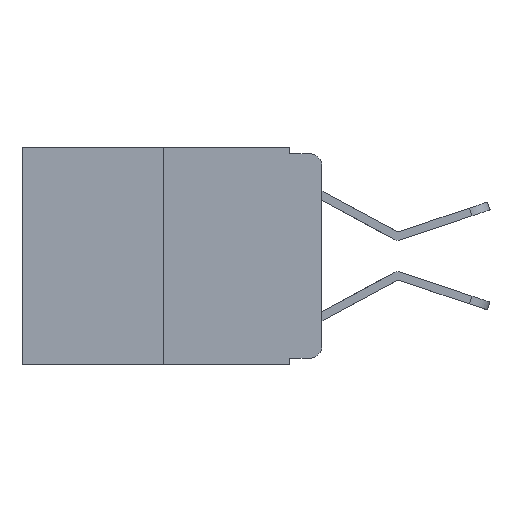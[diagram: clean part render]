
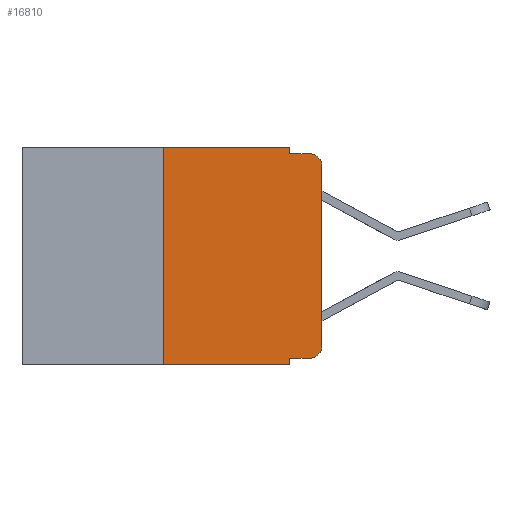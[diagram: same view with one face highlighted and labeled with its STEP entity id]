
A CAD part, left-side view. The second image highlights one B-rep face of the part: STEP entity #16810.
In plain terms, the highlighted planar face has unit normal (-1, 0, 0).
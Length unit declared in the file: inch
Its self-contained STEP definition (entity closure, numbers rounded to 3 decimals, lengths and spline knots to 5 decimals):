
#11 = EDGE_CURVE ( 'NONE', #2553, #739, #17145, .T. ) ;
#64 = ORIENTED_EDGE ( 'NONE', *, *, #16250, .F. ) ;
#450 = EDGE_CURVE ( 'NONE', #16306, #8936, #7758, .T. ) ;
#457 = CARTESIAN_POINT ( 'NONE',  ( 0., 0.02, -0.333 ) ) ;
#739 = VERTEX_POINT ( 'NONE', #10599 ) ;
#874 = CARTESIAN_POINT ( 'NONE',  ( 0., 0.473, -0.343 ) ) ;
#1337 = DIRECTION ( 'NONE',  ( 0., 0., 1. ) ) ;
#1581 = CARTESIAN_POINT ( 'NONE',  ( 0., 0.02, -0.313 ) ) ;
#1829 = EDGE_CURVE ( 'NONE', #11081, #2553, #3746, .T. ) ;
#2377 = PLANE ( 'NONE',  #7159 ) ;
#2470 = CARTESIAN_POINT ( 'NONE',  ( 0., 0.25, -0.343 ) ) ;
#2553 = VERTEX_POINT ( 'NONE', #6418 ) ;
#2650 = DIRECTION ( 'NONE',  ( 0., -1., 0. ) ) ;
#2667 = DIRECTION ( 'NONE',  ( 0., 0., -1. ) ) ;
#2817 = VERTEX_POINT ( 'NONE', #11243 ) ;
#3162 = VERTEX_POINT ( 'NONE', #4280 ) ;
#3557 = VERTEX_POINT ( 'NONE', #457 ) ;
#3746 = LINE ( 'NONE', #15966, #10415 ) ;
#3912 = CARTESIAN_POINT ( 'NONE',  ( 0., 0.473, 0. ) ) ;
#3955 = DIRECTION ( 'NONE',  ( 0., 0., -1. ) ) ;
#4280 = CARTESIAN_POINT ( 'NONE',  ( 0., 0.051, -0.343 ) ) ;
#4522 = VECTOR ( 'NONE', #1337, 39.37008 ) ;
#4531 = ORIENTED_EDGE ( 'NONE', *, *, #12968, .T. ) ;
#4738 = CIRCLE ( 'NONE', #11018, 0.02 ) ;
#5522 = CARTESIAN_POINT ( 'NONE',  ( 0., 0.051, 0. ) ) ;
#5604 = CARTESIAN_POINT ( 'NONE',  ( 0., 0., -0.313 ) ) ;
#5873 = DIRECTION ( 'NONE',  ( 0., 0., -1. ) ) ;
#5880 = DIRECTION ( 'NONE',  ( 0., 0., 1. ) ) ;
#5907 = DIRECTION ( 'NONE',  ( -1., 0., 0. ) ) ;
#6418 = CARTESIAN_POINT ( 'NONE',  ( 0., 0., -0.03 ) ) ;
#6440 = VECTOR ( 'NONE', #13638, 39.37008 ) ;
#6793 = EDGE_CURVE ( 'NONE', #2817, #3557, #14821, .T. ) ;
#6805 = ORIENTED_EDGE ( 'NONE', *, *, #10456, .F. ) ;
#7011 = EDGE_CURVE ( 'NONE', #8936, #14235, #13472, .T. ) ;
#7159 = AXIS2_PLACEMENT_3D ( 'NONE', #14167, #12727, #3955 ) ;
#7430 = ORIENTED_EDGE ( 'NONE', *, *, #7011, .F. ) ;
#7619 = CARTESIAN_POINT ( 'NONE',  ( 0., 0.051, 0. ) ) ;
#7758 = LINE ( 'NONE', #3912, #12862 ) ;
#8413 = CARTESIAN_POINT ( 'NONE',  ( 0., 0.25, 0. ) ) ;
#8647 = VECTOR ( 'NONE', #9802, 39.37008 ) ;
#8850 = CARTESIAN_POINT ( 'NONE',  ( 0., 0.25, 0. ) ) ;
#8936 = VERTEX_POINT ( 'NONE', #16142 ) ;
#8995 = ORIENTED_EDGE ( 'NONE', *, *, #450, .F. ) ;
#9296 = ORIENTED_EDGE ( 'NONE', *, *, #6793, .T. ) ;
#9513 = FACE_OUTER_BOUND ( 'NONE', #14394, .T. ) ;
#9802 = DIRECTION ( 'NONE',  ( 0., -1., 0. ) ) ;
#9856 = ORIENTED_EDGE ( 'NONE', *, *, #14492, .F. ) ;
#10194 = DIRECTION ( 'NONE',  ( 0., 0., -1. ) ) ;
#10196 = VECTOR ( 'NONE', #2667, 39.37008 ) ;
#10212 = VECTOR ( 'NONE', #10510, 39.37008 ) ;
#10415 = VECTOR ( 'NONE', #5880, 39.37008 ) ;
#10456 = EDGE_CURVE ( 'NONE', #16120, #16306, #14461, .T. ) ;
#10510 = DIRECTION ( 'NONE',  ( 0., -1., 0. ) ) ;
#10579 = EDGE_CURVE ( 'NONE', #3557, #11081, #4738, .T. ) ;
#10599 = CARTESIAN_POINT ( 'NONE',  ( 0., 0.02, -0.01 ) ) ;
#10630 = ORIENTED_EDGE ( 'NONE', *, *, #1829, .T. ) ;
#11018 = AXIS2_PLACEMENT_3D ( 'NONE', #1581, #11628, #5873 ) ;
#11081 = VERTEX_POINT ( 'NONE', #5604 ) ;
#11243 = CARTESIAN_POINT ( 'NONE',  ( 0., 0.051, -0.333 ) ) ;
#11628 = DIRECTION ( 'NONE',  ( -1., 0., 0. ) ) ;
#12258 = AXIS2_PLACEMENT_3D ( 'NONE', #12940, #5907, #10194 ) ;
#12681 = CARTESIAN_POINT ( 'NONE',  ( 0., 0.051, -0.01 ) ) ;
#12727 = DIRECTION ( 'NONE',  ( 1., 0., 0. ) ) ;
#12862 = VECTOR ( 'NONE', #2650, 39.37008 ) ;
#12940 = CARTESIAN_POINT ( 'NONE',  ( 0., 0.02, -0.03 ) ) ;
#12968 = EDGE_CURVE ( 'NONE', #16120, #3162, #15514, .T. ) ;
#13472 = LINE ( 'NONE', #5522, #10196 ) ;
#13638 = DIRECTION ( 'NONE',  ( 0., -1., 0. ) ) ;
#14063 = CARTESIAN_POINT ( 'NONE',  ( 0., 0.051, -0.01 ) ) ;
#14167 = CARTESIAN_POINT ( 'NONE',  ( 0., 0.473, 0. ) ) ;
#14235 = VERTEX_POINT ( 'NONE', #12681 ) ;
#14394 = EDGE_LOOP ( 'NONE', ( #10630, #17548, #64, #7430, #8995, #6805, #4531, #9856, #9296, #15928 ) ) ;
#14461 = LINE ( 'NONE', #8413, #4522 ) ;
#14492 = EDGE_CURVE ( 'NONE', #2817, #3162, #17781, .T. ) ;
#14603 = LINE ( 'NONE', #14063, #8647 ) ;
#14821 = LINE ( 'NONE', #18043, #10212 ) ;
#15341 = VECTOR ( 'NONE', #16050, 39.37008 ) ;
#15514 = LINE ( 'NONE', #874, #6440 ) ;
#15928 = ORIENTED_EDGE ( 'NONE', *, *, #10579, .T. ) ;
#15966 = CARTESIAN_POINT ( 'NONE',  ( 0., 0., 0. ) ) ;
#16050 = DIRECTION ( 'NONE',  ( 0., 0., -1. ) ) ;
#16120 = VERTEX_POINT ( 'NONE', #2470 ) ;
#16142 = CARTESIAN_POINT ( 'NONE',  ( 0., 0.051, 0. ) ) ;
#16250 = EDGE_CURVE ( 'NONE', #14235, #739, #14603, .T. ) ;
#16306 = VERTEX_POINT ( 'NONE', #8850 ) ;
#16810 = ADVANCED_FACE ( 'NONE', ( #9513 ), #2377, .F. ) ;
#17145 = CIRCLE ( 'NONE', #12258, 0.02 ) ;
#17548 = ORIENTED_EDGE ( 'NONE', *, *, #11, .T. ) ;
#17781 = LINE ( 'NONE', #7619, #15341 ) ;
#18043 = CARTESIAN_POINT ( 'NONE',  ( 0., 0.051, -0.333 ) ) ;
